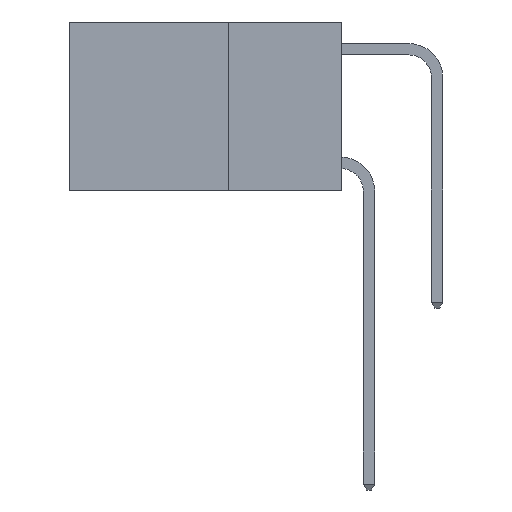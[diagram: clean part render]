
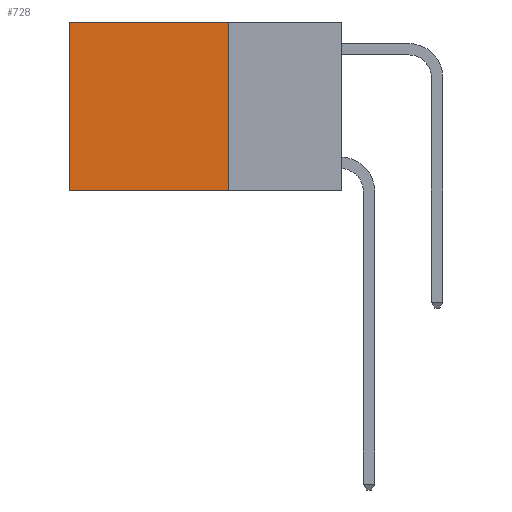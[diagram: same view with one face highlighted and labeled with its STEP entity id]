
A CAD part, left-side view. The second image highlights one B-rep face of the part: STEP entity #728.
In plain terms, the highlighted planar face has unit normal (-1, 0, 0).
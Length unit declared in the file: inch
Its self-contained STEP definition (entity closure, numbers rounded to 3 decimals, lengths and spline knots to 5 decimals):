
#27 = CARTESIAN_POINT ( 'NONE',  ( 0.2625, 0.25, 0. ) ) ;
#114 = ORIENTED_EDGE ( 'NONE', *, *, #11637, .T. ) ;
#244 = EDGE_CURVE ( 'NONE', #7081, #1127, #1385, .T. ) ;
#728 = ADVANCED_FACE ( 'NONE', ( #2970 ), #2540, .F. ) ;
#1127 = VERTEX_POINT ( 'NONE', #3071 ) ;
#1249 = EDGE_LOOP ( 'NONE', ( #7810, #6931, #10697, #114 ) ) ;
#1385 = LINE ( 'NONE', #6366, #8610 ) ;
#2321 = CARTESIAN_POINT ( 'NONE',  ( 0.2625, 0.6, 0. ) ) ;
#2513 = AXIS2_PLACEMENT_3D ( 'NONE', #11923, #3043, #6001 ) ;
#2540 = PLANE ( 'NONE',  #2513 ) ;
#2658 = VERTEX_POINT ( 'NONE', #9200 ) ;
#2837 = CARTESIAN_POINT ( 'NONE',  ( 0.2625, 0.25, 0. ) ) ;
#2970 = FACE_OUTER_BOUND ( 'NONE', #1249, .T. ) ;
#3043 = DIRECTION ( 'NONE',  ( 1., 0., 0. ) ) ;
#3071 = CARTESIAN_POINT ( 'NONE',  ( 0.2625, 0.6, -0.37 ) ) ;
#3166 = DIRECTION ( 'NONE',  ( 0., 1., 0. ) ) ;
#3352 = VECTOR ( 'NONE', #3166, 39.37008 ) ;
#3511 = LINE ( 'NONE', #2837, #8433 ) ;
#3841 = LINE ( 'NONE', #9962, #6002 ) ;
#3950 = LINE ( 'NONE', #27, #3352 ) ;
#4072 = EDGE_CURVE ( 'NONE', #5567, #1127, #3841, .T. ) ;
#5567 = VERTEX_POINT ( 'NONE', #2321 ) ;
#5642 = DIRECTION ( 'NONE',  ( 0., 0., -1. ) ) ;
#5984 = EDGE_CURVE ( 'NONE', #2658, #7081, #3511, .T. ) ;
#6001 = DIRECTION ( 'NONE',  ( 0., 0., -1. ) ) ;
#6002 = VECTOR ( 'NONE', #9028, 39.37008 ) ;
#6366 = CARTESIAN_POINT ( 'NONE',  ( 0.2625, 0.25, -0.37 ) ) ;
#6931 = ORIENTED_EDGE ( 'NONE', *, *, #244, .F. ) ;
#7081 = VERTEX_POINT ( 'NONE', #11358 ) ;
#7810 = ORIENTED_EDGE ( 'NONE', *, *, #4072, .T. ) ;
#8383 = DIRECTION ( 'NONE',  ( 0., 1., 0. ) ) ;
#8433 = VECTOR ( 'NONE', #5642, 39.37008 ) ;
#8610 = VECTOR ( 'NONE', #8383, 39.37008 ) ;
#9028 = DIRECTION ( 'NONE',  ( 0., 0., -1. ) ) ;
#9200 = CARTESIAN_POINT ( 'NONE',  ( 0.2625, 0.25, 0. ) ) ;
#9962 = CARTESIAN_POINT ( 'NONE',  ( 0.2625, 0.6, 0. ) ) ;
#10697 = ORIENTED_EDGE ( 'NONE', *, *, #5984, .F. ) ;
#11358 = CARTESIAN_POINT ( 'NONE',  ( 0.2625, 0.25, -0.37 ) ) ;
#11637 = EDGE_CURVE ( 'NONE', #2658, #5567, #3950, .T. ) ;
#11923 = CARTESIAN_POINT ( 'NONE',  ( 0.2625, 0.25, 0. ) ) ;
